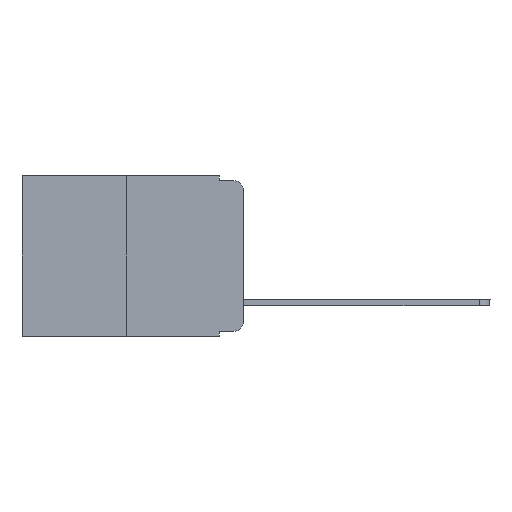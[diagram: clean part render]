
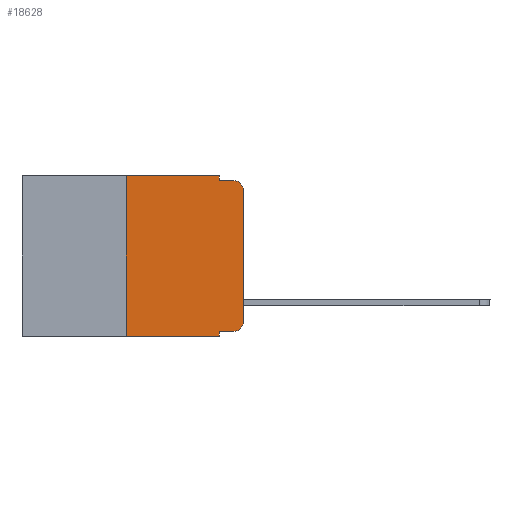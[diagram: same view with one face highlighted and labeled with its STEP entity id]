
A CAD part, left-side view. The second image highlights one B-rep face of the part: STEP entity #18628.
In plain terms, the highlighted planar face has unit normal (-1, 0, 0).
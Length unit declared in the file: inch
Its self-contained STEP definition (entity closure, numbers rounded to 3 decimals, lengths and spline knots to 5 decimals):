
#333 = EDGE_CURVE ( 'NONE', #11157, #6761, #15551, .T. ) ;
#526 = AXIS2_PLACEMENT_3D ( 'NONE', #11398, #9567, #14274 ) ;
#1239 = CARTESIAN_POINT ( 'NONE',  ( 0., 0.051, -0.333 ) ) ;
#1331 = VERTEX_POINT ( 'NONE', #11169 ) ;
#1737 = CARTESIAN_POINT ( 'NONE',  ( 0., 0., -0.313 ) ) ;
#1754 = CARTESIAN_POINT ( 'NONE',  ( 0., 0.051, -0.343 ) ) ;
#1755 = VECTOR ( 'NONE', #12156, 39.37008 ) ;
#1817 = AXIS2_PLACEMENT_3D ( 'NONE', #18397, #18195, #5701 ) ;
#1998 = CARTESIAN_POINT ( 'NONE',  ( 0., 0., -0.03 ) ) ;
#2204 = LINE ( 'NONE', #14745, #20043 ) ;
#2225 = ORIENTED_EDGE ( 'NONE', *, *, #8096, .F. ) ;
#2466 = EDGE_CURVE ( 'NONE', #6295, #11157, #2204, .T. ) ;
#2517 = AXIS2_PLACEMENT_3D ( 'NONE', #8897, #15146, #14939 ) ;
#3172 = VERTEX_POINT ( 'NONE', #14058 ) ;
#3810 = DIRECTION ( 'NONE',  ( 0., 0., -1. ) ) ;
#4026 = ORIENTED_EDGE ( 'NONE', *, *, #5898, .F. ) ;
#4208 = EDGE_CURVE ( 'NONE', #3172, #10911, #5892, .T. ) ;
#4280 = EDGE_CURVE ( 'NONE', #1331, #4396, #15578, .T. ) ;
#4396 = VERTEX_POINT ( 'NONE', #1754 ) ;
#4741 = LINE ( 'NONE', #18373, #6975 ) ;
#4763 = VECTOR ( 'NONE', #11631, 39.37008 ) ;
#5142 = CIRCLE ( 'NONE', #526, 0.02 ) ;
#5701 = DIRECTION ( 'NONE',  ( 0., 0., -1. ) ) ;
#5892 = LINE ( 'NONE', #1239, #1755 ) ;
#5898 = EDGE_CURVE ( 'NONE', #11593, #6295, #4741, .T. ) ;
#6250 = DIRECTION ( 'NONE',  ( 0., -1., 0. ) ) ;
#6295 = VERTEX_POINT ( 'NONE', #11244 ) ;
#6561 = CARTESIAN_POINT ( 'NONE',  ( 0., 0.051, -0.01 ) ) ;
#6715 = ORIENTED_EDGE ( 'NONE', *, *, #15247, .F. ) ;
#6761 = VERTEX_POINT ( 'NONE', #9864 ) ;
#6975 = VECTOR ( 'NONE', #11000, 39.37008 ) ;
#7133 = ORIENTED_EDGE ( 'NONE', *, *, #4208, .T. ) ;
#7873 = CARTESIAN_POINT ( 'NONE',  ( 0., 0.25, 0. ) ) ;
#8096 = EDGE_CURVE ( 'NONE', #1331, #11593, #10292, .T. ) ;
#8485 = EDGE_CURVE ( 'NONE', #10803, #18692, #13216, .T. ) ;
#8486 = VECTOR ( 'NONE', #6250, 39.37008 ) ;
#8693 = FACE_OUTER_BOUND ( 'NONE', #17137, .T. ) ;
#8897 = CARTESIAN_POINT ( 'NONE',  ( 0., 0.473, 0. ) ) ;
#9073 = EDGE_CURVE ( 'NONE', #10911, #10803, #19511, .T. ) ;
#9138 = ORIENTED_EDGE ( 'NONE', *, *, #333, .F. ) ;
#9567 = DIRECTION ( 'NONE',  ( -1., 0., 0. ) ) ;
#9756 = EDGE_CURVE ( 'NONE', #18692, #6761, #5142, .T. ) ;
#9864 = CARTESIAN_POINT ( 'NONE',  ( 0., 0.02, -0.01 ) ) ;
#10024 = PLANE ( 'NONE',  #2517 ) ;
#10292 = LINE ( 'NONE', #16527, #4763 ) ;
#10803 = VERTEX_POINT ( 'NONE', #1737 ) ;
#10911 = VERTEX_POINT ( 'NONE', #13447 ) ;
#11000 = DIRECTION ( 'NONE',  ( 0., -1., 0. ) ) ;
#11157 = VERTEX_POINT ( 'NONE', #6561 ) ;
#11169 = CARTESIAN_POINT ( 'NONE',  ( 0., 0.25, -0.343 ) ) ;
#11244 = CARTESIAN_POINT ( 'NONE',  ( 0., 0.051, 0. ) ) ;
#11398 = CARTESIAN_POINT ( 'NONE',  ( 0., 0.02, -0.03 ) ) ;
#11593 = VERTEX_POINT ( 'NONE', #7873 ) ;
#11631 = DIRECTION ( 'NONE',  ( 0., 0., 1. ) ) ;
#12156 = DIRECTION ( 'NONE',  ( 0., -1., 0. ) ) ;
#12673 = ORIENTED_EDGE ( 'NONE', *, *, #9756, .T. ) ;
#12989 = ORIENTED_EDGE ( 'NONE', *, *, #4280, .T. ) ;
#13040 = LINE ( 'NONE', #14793, #19657 ) ;
#13216 = LINE ( 'NONE', #19450, #19164 ) ;
#13447 = CARTESIAN_POINT ( 'NONE',  ( 0., 0.02, -0.333 ) ) ;
#14058 = CARTESIAN_POINT ( 'NONE',  ( 0., 0.051, -0.333 ) ) ;
#14274 = DIRECTION ( 'NONE',  ( 0., 0., -1. ) ) ;
#14583 = ORIENTED_EDGE ( 'NONE', *, *, #8485, .T. ) ;
#14745 = CARTESIAN_POINT ( 'NONE',  ( 0., 0.051, 0. ) ) ;
#14793 = CARTESIAN_POINT ( 'NONE',  ( 0., 0.051, 0. ) ) ;
#14939 = DIRECTION ( 'NONE',  ( 0., 0., -1. ) ) ;
#15146 = DIRECTION ( 'NONE',  ( 1., 0., 0. ) ) ;
#15247 = EDGE_CURVE ( 'NONE', #3172, #4396, #13040, .T. ) ;
#15345 = CARTESIAN_POINT ( 'NONE',  ( 0., 0.051, -0.01 ) ) ;
#15551 = LINE ( 'NONE', #15345, #17685 ) ;
#15578 = LINE ( 'NONE', #20282, #8486 ) ;
#16527 = CARTESIAN_POINT ( 'NONE',  ( 0., 0.25, 0. ) ) ;
#17137 = EDGE_LOOP ( 'NONE', ( #14583, #12673, #9138, #17666, #4026, #2225, #12989, #6715, #7133, #19081 ) ) ;
#17666 = ORIENTED_EDGE ( 'NONE', *, *, #2466, .F. ) ;
#17685 = VECTOR ( 'NONE', #19945, 39.37008 ) ;
#17713 = DIRECTION ( 'NONE',  ( 0., 0., 1. ) ) ;
#18195 = DIRECTION ( 'NONE',  ( -1., 0., 0. ) ) ;
#18373 = CARTESIAN_POINT ( 'NONE',  ( 0., 0.473, 0. ) ) ;
#18397 = CARTESIAN_POINT ( 'NONE',  ( 0., 0.02, -0.313 ) ) ;
#18628 = ADVANCED_FACE ( 'NONE', ( #8693 ), #10024, .F. ) ;
#18692 = VERTEX_POINT ( 'NONE', #1998 ) ;
#19081 = ORIENTED_EDGE ( 'NONE', *, *, #9073, .T. ) ;
#19164 = VECTOR ( 'NONE', #17713, 39.37008 ) ;
#19237 = DIRECTION ( 'NONE',  ( 0., 0., -1. ) ) ;
#19450 = CARTESIAN_POINT ( 'NONE',  ( 0., 0., 0. ) ) ;
#19511 = CIRCLE ( 'NONE', #1817, 0.02 ) ;
#19657 = VECTOR ( 'NONE', #3810, 39.37008 ) ;
#19945 = DIRECTION ( 'NONE',  ( 0., -1., 0. ) ) ;
#20043 = VECTOR ( 'NONE', #19237, 39.37008 ) ;
#20282 = CARTESIAN_POINT ( 'NONE',  ( 0., 0.473, -0.343 ) ) ;
